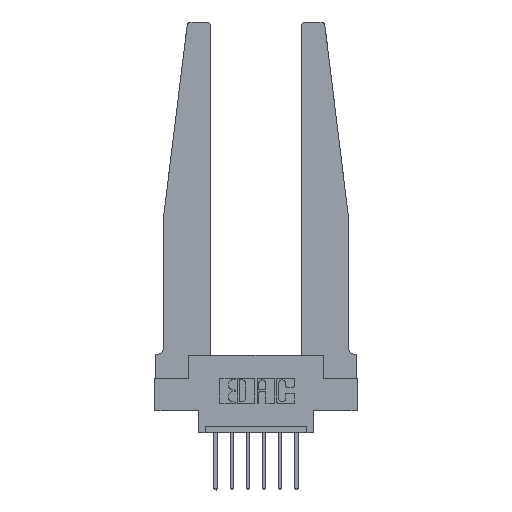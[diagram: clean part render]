
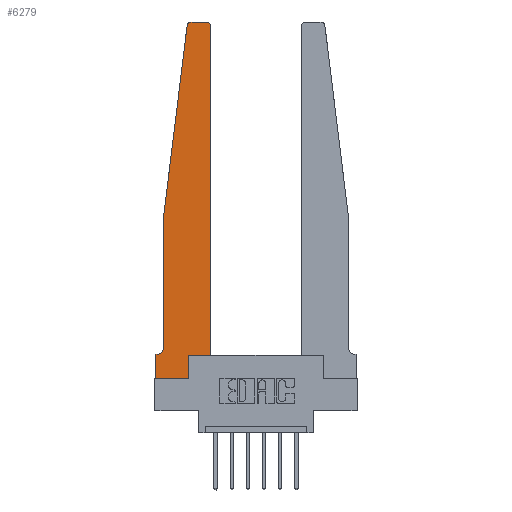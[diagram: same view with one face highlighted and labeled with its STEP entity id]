
A CAD part, top view. The second image highlights one B-rep face of the part: STEP entity #6279.
In plain terms, the highlighted planar face has unit normal (0, 0, 1).
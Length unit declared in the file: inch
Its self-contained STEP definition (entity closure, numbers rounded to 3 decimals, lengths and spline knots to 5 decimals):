
#329 = EDGE_CURVE ( 'NONE', #9085, #2658, #11552, .T. ) ;
#550 = DIRECTION ( 'NONE',  ( 0., -1., 0. ) ) ;
#970 = EDGE_CURVE ( 'NONE', #1491, #6536, #12166, .T. ) ;
#1067 = DIRECTION ( 'NONE',  ( 0., 0., -1. ) ) ;
#1120 = LINE ( 'NONE', #9688, #4663 ) ;
#1491 = VERTEX_POINT ( 'NONE', #7244 ) ;
#1501 = EDGE_CURVE ( 'NONE', #10224, #10375, #10633, .T. ) ;
#1507 = CARTESIAN_POINT ( 'NONE',  ( 0.395, 2.72, 0.37 ) ) ;
#1520 = EDGE_CURVE ( 'NONE', #13070, #2331, #2715, .T. ) ;
#1766 = EDGE_CURVE ( 'NONE', #10375, #3249, #9111, .T. ) ;
#1958 = ORIENTED_EDGE ( 'NONE', *, *, #1520, .T. ) ;
#2331 = VERTEX_POINT ( 'NONE', #9591 ) ;
#2349 = ORIENTED_EDGE ( 'NONE', *, *, #1766, .T. ) ;
#2374 = EDGE_LOOP ( 'NONE', ( #7984, #2349, #7942, #10132, #1958, #4845, #12025, #2896, #11497, #4480, #10010, #10988 ) ) ;
#2375 = VECTOR ( 'NONE', #550, 39.37008 ) ;
#2658 = VERTEX_POINT ( 'NONE', #10343 ) ;
#2715 = CIRCLE ( 'NONE', #10567, 0.05 ) ;
#2750 = DIRECTION ( 'NONE',  ( 0., 0., 1. ) ) ;
#2869 = PLANE ( 'NONE',  #10818 ) ;
#2896 = ORIENTED_EDGE ( 'NONE', *, *, #3797, .T. ) ;
#2902 = CARTESIAN_POINT ( 'NONE',  ( 0.25, 2.75, 0.37 ) ) ;
#3186 = CARTESIAN_POINT ( 'NONE',  ( 0.425, 2.72, 0.37 ) ) ;
#3249 = VERTEX_POINT ( 'NONE', #5346 ) ;
#3306 = DIRECTION ( 'NONE',  ( -1., 0., 0. ) ) ;
#3475 = EDGE_CURVE ( 'NONE', #2331, #9085, #1120, .T. ) ;
#3493 = DIRECTION ( 'NONE',  ( 0., 1., 0. ) ) ;
#3797 = EDGE_CURVE ( 'NONE', #2658, #1491, #4055, .T. ) ;
#3917 = CARTESIAN_POINT ( 'NONE',  ( 0.425, 0.18, 0.37 ) ) ;
#4048 = EDGE_CURVE ( 'NONE', #3249, #4066, #10641, .T. ) ;
#4055 = LINE ( 'NONE', #5235, #4235 ) ;
#4066 = VERTEX_POINT ( 'NONE', #4258 ) ;
#4081 = CARTESIAN_POINT ( 'NONE',  ( 0.065, 1.25, 0.37 ) ) ;
#4180 = EDGE_CURVE ( 'NONE', #6536, #10710, #6966, .T. ) ;
#4235 = VECTOR ( 'NONE', #11671, 39.37008 ) ;
#4258 = CARTESIAN_POINT ( 'NONE',  ( 0.065, 1.25, 0.37 ) ) ;
#4480 = ORIENTED_EDGE ( 'NONE', *, *, #4180, .T. ) ;
#4663 = VECTOR ( 'NONE', #3306, 39.37008 ) ;
#4722 = DIRECTION ( 'NONE',  ( 0., -1., 0. ) ) ;
#4745 = CARTESIAN_POINT ( 'NONE',  ( 0.2605, 0.18, 0.37 ) ) ;
#4845 = ORIENTED_EDGE ( 'NONE', *, *, #3475, .T. ) ;
#4850 = DIRECTION ( 'NONE',  ( 1., 0., 0. ) ) ;
#4901 = CARTESIAN_POINT ( 'NONE',  ( 0., 0.1875, 0.37 ) ) ;
#5235 = CARTESIAN_POINT ( 'NONE',  ( 0., 0., 0.37 ) ) ;
#5299 = CARTESIAN_POINT ( 'NONE',  ( 0.065, 1.25, 0.37 ) ) ;
#5346 = CARTESIAN_POINT ( 'NONE',  ( 0.24675, 2.72367, 0.37 ) ) ;
#5912 = CARTESIAN_POINT ( 'NONE',  ( 0.27653, 2.72, 0.37 ) ) ;
#5923 = DIRECTION ( 'NONE',  ( 1., 0., 0. ) ) ;
#5931 = EDGE_CURVE ( 'NONE', #10710, #11306, #10682, .T. ) ;
#5961 = VECTOR ( 'NONE', #11772, 39.37008 ) ;
#6279 = ADVANCED_FACE ( 'NONE', ( #10241 ), #2869, .T. ) ;
#6422 = DIRECTION ( 'NONE',  ( -1., 0., 0. ) ) ;
#6536 = VERTEX_POINT ( 'NONE', #4745 ) ;
#6904 = CARTESIAN_POINT ( 'NONE',  ( 0., 0., 0.37 ) ) ;
#6966 = LINE ( 'NONE', #11216, #9292 ) ;
#7244 = CARTESIAN_POINT ( 'NONE',  ( 0.2605, 0., 0.37 ) ) ;
#7565 = VECTOR ( 'NONE', #4722, 39.37008 ) ;
#7748 = AXIS2_PLACEMENT_3D ( 'NONE', #1507, #9023, #13333 ) ;
#7942 = ORIENTED_EDGE ( 'NONE', *, *, #4048, .T. ) ;
#7984 = ORIENTED_EDGE ( 'NONE', *, *, #1501, .T. ) ;
#8078 = LINE ( 'NONE', #4081, #2375 ) ;
#8383 = DIRECTION ( 'NONE',  ( -1., 0., 0. ) ) ;
#8626 = VECTOR ( 'NONE', #9584, 39.37008 ) ;
#8797 = VECTOR ( 'NONE', #3493, 39.37008 ) ;
#8829 = CARTESIAN_POINT ( 'NONE',  ( 0.2605, 0.18, 0.37 ) ) ;
#9023 = DIRECTION ( 'NONE',  ( 0., 0., 1. ) ) ;
#9065 = CARTESIAN_POINT ( 'NONE',  ( 0., 0.1875, 0.37 ) ) ;
#9085 = VERTEX_POINT ( 'NONE', #9065 ) ;
#9111 = CIRCLE ( 'NONE', #10926, 0.03 ) ;
#9186 = DIRECTION ( 'NONE',  ( 0., 0., 1. ) ) ;
#9292 = VECTOR ( 'NONE', #5923, 39.37008 ) ;
#9298 = EDGE_CURVE ( 'NONE', #11306, #10224, #12503, .T. ) ;
#9584 = DIRECTION ( 'NONE',  ( -0.122, -0.992, 0. ) ) ;
#9591 = CARTESIAN_POINT ( 'NONE',  ( 0.015, 0.1875, 0.37 ) ) ;
#9688 = CARTESIAN_POINT ( 'NONE',  ( 0.065, 0.1875, 0.37 ) ) ;
#10010 = ORIENTED_EDGE ( 'NONE', *, *, #5931, .T. ) ;
#10132 = ORIENTED_EDGE ( 'NONE', *, *, #10155, .T. ) ;
#10155 = EDGE_CURVE ( 'NONE', #4066, #13070, #8078, .T. ) ;
#10178 = CARTESIAN_POINT ( 'NONE',  ( 0.395, 2.75, 0.37 ) ) ;
#10224 = VERTEX_POINT ( 'NONE', #10178 ) ;
#10241 = FACE_OUTER_BOUND ( 'NONE', #2374, .T. ) ;
#10343 = CARTESIAN_POINT ( 'NONE',  ( 0., 0., 0.37 ) ) ;
#10375 = VERTEX_POINT ( 'NONE', #11767 ) ;
#10567 = AXIS2_PLACEMENT_3D ( 'NONE', #13882, #1067, #8383 ) ;
#10633 = LINE ( 'NONE', #2902, #12857 ) ;
#10641 = LINE ( 'NONE', #5299, #8626 ) ;
#10682 = LINE ( 'NONE', #12834, #5961 ) ;
#10710 = VERTEX_POINT ( 'NONE', #3917 ) ;
#10818 = AXIS2_PLACEMENT_3D ( 'NONE', #4901, #9186, #13490 ) ;
#10833 = CARTESIAN_POINT ( 'NONE',  ( 0.065, 0.2375, 0.37 ) ) ;
#10926 = AXIS2_PLACEMENT_3D ( 'NONE', #5912, #2750, #4850 ) ;
#10988 = ORIENTED_EDGE ( 'NONE', *, *, #9298, .T. ) ;
#11216 = CARTESIAN_POINT ( 'NONE',  ( 0.425, 0.18, 0.37 ) ) ;
#11306 = VERTEX_POINT ( 'NONE', #3186 ) ;
#11497 = ORIENTED_EDGE ( 'NONE', *, *, #970, .T. ) ;
#11552 = LINE ( 'NONE', #6904, #7565 ) ;
#11671 = DIRECTION ( 'NONE',  ( 1., 0., 0. ) ) ;
#11767 = CARTESIAN_POINT ( 'NONE',  ( 0.27653, 2.75, 0.37 ) ) ;
#11772 = DIRECTION ( 'NONE',  ( 0., 1., 0. ) ) ;
#12025 = ORIENTED_EDGE ( 'NONE', *, *, #329, .T. ) ;
#12166 = LINE ( 'NONE', #8829, #8797 ) ;
#12503 = CIRCLE ( 'NONE', #7748, 0.03 ) ;
#12834 = CARTESIAN_POINT ( 'NONE',  ( 0.425, 0.18, 0.37 ) ) ;
#12857 = VECTOR ( 'NONE', #6422, 39.37008 ) ;
#13070 = VERTEX_POINT ( 'NONE', #10833 ) ;
#13333 = DIRECTION ( 'NONE',  ( 1., 0., 0. ) ) ;
#13490 = DIRECTION ( 'NONE',  ( 1., 0., 0. ) ) ;
#13882 = CARTESIAN_POINT ( 'NONE',  ( 0.015, 0.2375, 0.37 ) ) ;
